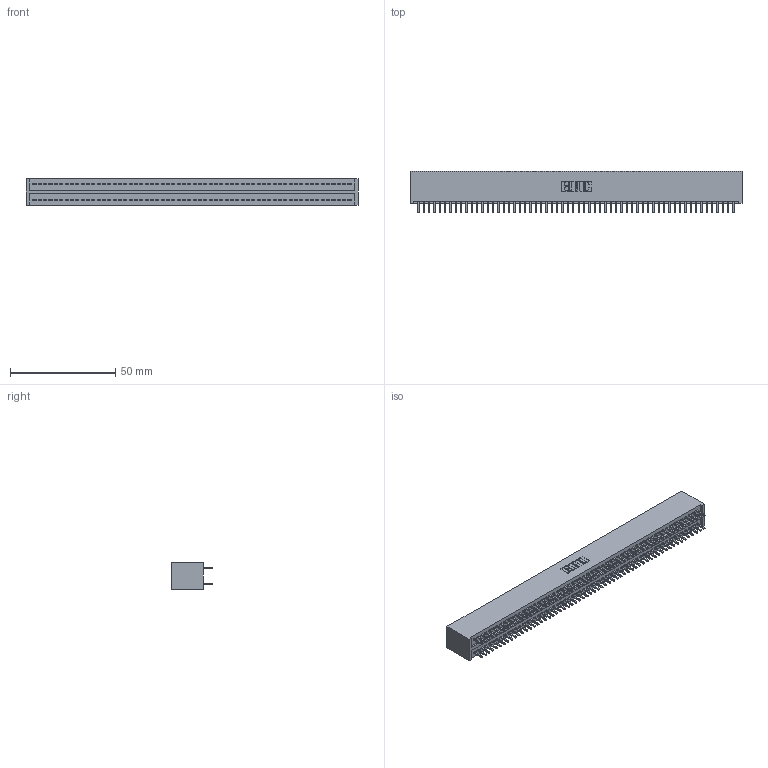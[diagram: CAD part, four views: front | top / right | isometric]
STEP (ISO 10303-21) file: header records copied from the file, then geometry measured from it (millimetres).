
FILE_DESCRIPTION (( 'STEP AP203' ), '1' );
FILE_NAME ('325-120-520-201.STEP', '2020-02-25T08:41:53', ( '' ), ( '' ), 'SwSTEP 2.0', 'SolidWorks 2016', '' );
FILE_SCHEMA (( 'CONFIG_CONTROL_DESIGN' ));
Length unit declared in the file: inch
Products named in the file (3): 325 Part_Lugless; 325-120-520-201; 325-292-001_325-293-120
Assembly tree (121 placements, depth 2):
  325-120-520-201
    325 Part_Lugless
    325-292-001_325-293-120  x120
Bounding box: 158.04 x 19.68 x 12.45 mm (x, y, z)
Volume: 21151.8 mm3; surface area: 26446.9 mm2
Topology: 121 solids, 121 shells, 6346 faces, 18887 edges, 12430 vertices
Faces by surface type: plane 4386, cylinder 1960
Entity records: 36013 total; most frequent: CARTESIAN_POINT 5946, ORIENTED_EDGE 5882, DIRECTION 5041, EDGE_CURVE 2941, LINE 2821, VECTOR 2821, VERTEX_POINT 1958, AXIS2_PLACEMENT_3D 1110
